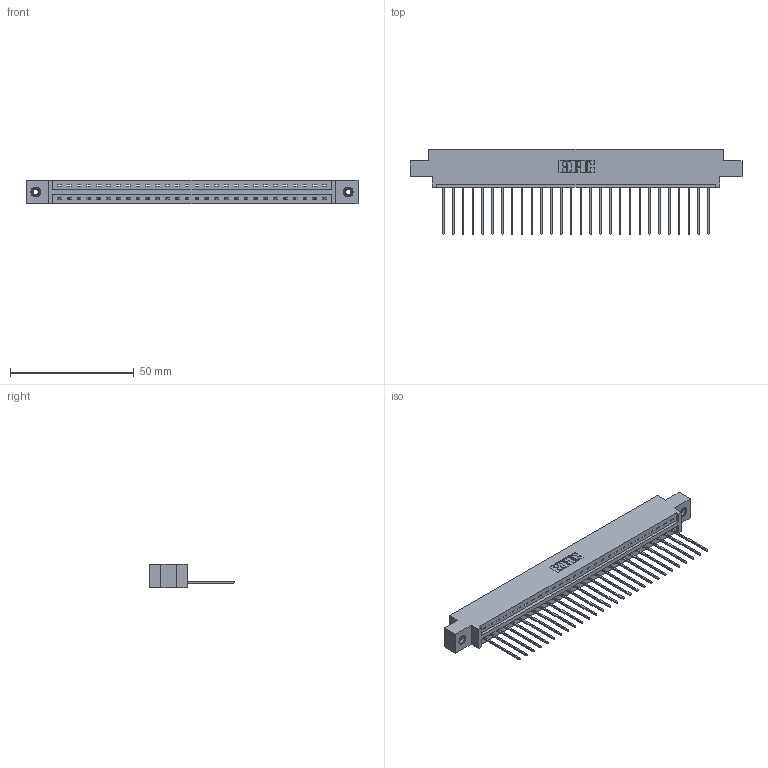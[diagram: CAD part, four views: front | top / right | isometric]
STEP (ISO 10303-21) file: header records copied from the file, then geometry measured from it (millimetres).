
FILE_DESCRIPTION (( 'STEP AP203' ), '1' );
FILE_NAME ('387-028-541-608.STEP', '2018-09-16T20:54:24', ( '' ), ( '' ), 'SwSTEP 2.0', 'SolidWorks 2016', '' );
FILE_SCHEMA (( 'CONFIG_CONTROL_DESIGN' ));
Length unit declared in the file: inch
Products named in the file (4): 337 Part_0.170 Offset - 0.156 Dia-TI; 345-292-001_345-293-141; 345-250-001_345-250-003-102; 387-028-541-608
Assembly tree (31 placements, depth 2):
  387-028-541-608
    337 Part_0.170 Offset - 0.156 Dia-TI
    345-292-001_345-293-141  x28
    345-250-001_345-250-003-102  x2
Bounding box: 133.96 x 34.3 x 9.4 mm (x, y, z)
Volume: 13716 mm3; surface area: 14790.3 mm2
Topology: 31 solids, 31 shells, 1914 faces, 5723 edges, 3770 vertices
Faces by surface type: plane 1394, cylinder 504, cone 12, torus 4
Entity records: 23960 total; most frequent: CARTESIAN_POINT 4153, ORIENTED_EDGE 4110, DIRECTION 3557, EDGE_CURVE 2055, LINE 1907, VECTOR 1907, VERTEX_POINT 1364, AXIS2_PLACEMENT_3D 825
